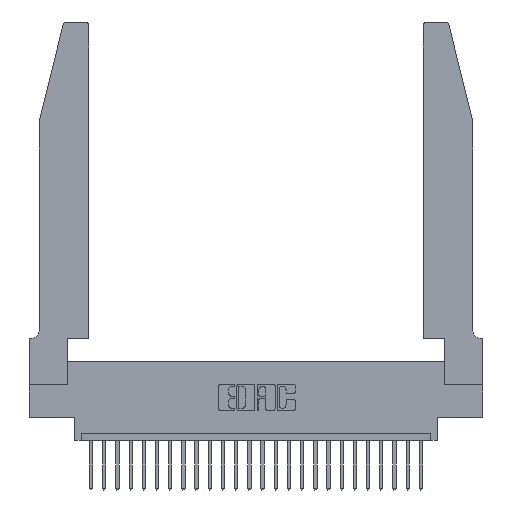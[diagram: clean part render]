
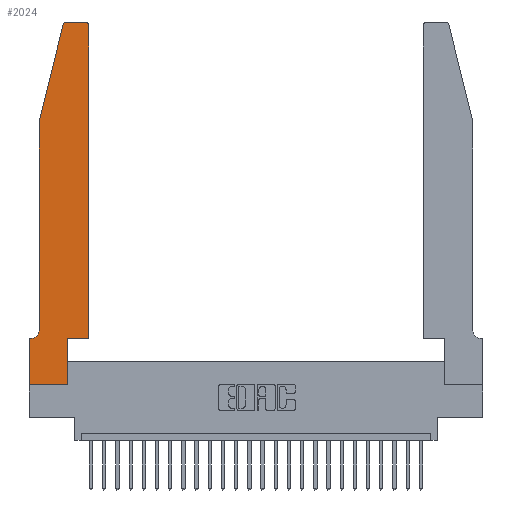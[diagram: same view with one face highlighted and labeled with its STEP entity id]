
A CAD part, top view. The second image highlights one B-rep face of the part: STEP entity #2024.
In plain terms, the highlighted planar face has unit normal (0, 0, 1).
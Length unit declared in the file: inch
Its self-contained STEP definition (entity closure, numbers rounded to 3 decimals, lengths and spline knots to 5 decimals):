
#787 = EDGE_CURVE ( 'NONE', #14174, #3340, #11736, .T. ) ;
#948 = DIRECTION ( 'NONE',  ( -1., 0., 0. ) ) ;
#1376 = DIRECTION ( 'NONE',  ( 1., 0., 0. ) ) ;
#1404 = VERTEX_POINT ( 'NONE', #18449 ) ;
#1429 = EDGE_CURVE ( 'NONE', #3409, #15677, #10569, .T. ) ;
#1465 = CIRCLE ( 'NONE', #21558, 0.07 ) ;
#1536 = DIRECTION ( 'NONE',  ( 0., -1., 0. ) ) ;
#2024 = ADVANCED_FACE ( 'NONE', ( #20470 ), #5938, .T. ) ;
#2081 = ORIENTED_EDGE ( 'NONE', *, *, #1429, .T. ) ;
#2490 = CARTESIAN_POINT ( 'NONE',  ( 0.2865, 0.35, 0.37 ) ) ;
#2954 = EDGE_CURVE ( 'NONE', #20707, #10282, #26242, .T. ) ;
#2961 = EDGE_CURVE ( 'NONE', #1404, #26402, #23984, .T. ) ;
#3164 = AXIS2_PLACEMENT_3D ( 'NONE', #8856, #6872, #21214 ) ;
#3340 = VERTEX_POINT ( 'NONE', #10819 ) ;
#3409 = VERTEX_POINT ( 'NONE', #19411 ) ;
#3444 = LINE ( 'NONE', #25226, #24611 ) ;
#3613 = EDGE_CURVE ( 'NONE', #10282, #20843, #3444, .T. ) ;
#3735 = ORIENTED_EDGE ( 'NONE', *, *, #4351, .T. ) ;
#3754 = VECTOR ( 'NONE', #24382, 39.37008 ) ;
#3763 = ORIENTED_EDGE ( 'NONE', *, *, #14501, .T. ) ;
#3949 = DIRECTION ( 'NONE',  ( 1., 0., 0. ) ) ;
#4347 = VERTEX_POINT ( 'NONE', #23082 ) ;
#4351 = EDGE_CURVE ( 'NONE', #20843, #3409, #5001, .T. ) ;
#4552 = DIRECTION ( 'NONE',  ( 0., 1., 0. ) ) ;
#5001 = LINE ( 'NONE', #21393, #19768 ) ;
#5045 = DIRECTION ( 'NONE',  ( -1., 0., 0. ) ) ;
#5938 = PLANE ( 'NONE',  #10742 ) ;
#6380 = CIRCLE ( 'NONE', #23471, 0.03 ) ;
#6781 = CARTESIAN_POINT ( 'NONE',  ( 0.0755, 0.35, 0.37 ) ) ;
#6872 = DIRECTION ( 'NONE',  ( 0., 0., 1. ) ) ;
#7204 = ORIENTED_EDGE ( 'NONE', *, *, #15792, .T. ) ;
#8226 = VECTOR ( 'NONE', #948, 39.37008 ) ;
#8350 = VERTEX_POINT ( 'NONE', #10346 ) ;
#8856 = CARTESIAN_POINT ( 'NONE',  ( 0.4205, 2.72, 0.37 ) ) ;
#10282 = VERTEX_POINT ( 'NONE', #19364 ) ;
#10346 = CARTESIAN_POINT ( 'NONE',  ( 0.284, 2.75, 0.37 ) ) ;
#10569 = LINE ( 'NONE', #2490, #11249 ) ;
#10742 = AXIS2_PLACEMENT_3D ( 'NONE', #16508, #18224, #3949 ) ;
#10819 = CARTESIAN_POINT ( 'NONE',  ( 0.0755, 0.42, 0.37 ) ) ;
#11159 = DIRECTION ( 'NONE',  ( 0., -1., 0. ) ) ;
#11249 = VECTOR ( 'NONE', #4552, 39.37008 ) ;
#11252 = CARTESIAN_POINT ( 'NONE',  ( 0.2865, 0.35, 0.37 ) ) ;
#11599 = DIRECTION ( 'NONE',  ( -0.239, -0.971, 0. ) ) ;
#11736 = LINE ( 'NONE', #19473, #17808 ) ;
#11814 = ORIENTED_EDGE ( 'NONE', *, *, #2961, .T. ) ;
#11885 = EDGE_CURVE ( 'NONE', #15677, #24329, #20150, .T. ) ;
#12162 = ORIENTED_EDGE ( 'NONE', *, *, #787, .T. ) ;
#12865 = CARTESIAN_POINT ( 'NONE',  ( 0.0055, 0.42, 0.37 ) ) ;
#13418 = VECTOR ( 'NONE', #11599, 39.37008 ) ;
#14174 = VERTEX_POINT ( 'NONE', #14208 ) ;
#14203 = EDGE_CURVE ( 'NONE', #3340, #20707, #1465, .T. ) ;
#14208 = CARTESIAN_POINT ( 'NONE',  ( 0.0755, 2., 0.37 ) ) ;
#14263 = VECTOR ( 'NONE', #21679, 39.37008 ) ;
#14501 = EDGE_CURVE ( 'NONE', #26402, #8350, #15268, .T. ) ;
#14611 = VECTOR ( 'NONE', #15788, 39.37008 ) ;
#14901 = DIRECTION ( 'NONE',  ( 0., 0., -1. ) ) ;
#15070 = ORIENTED_EDGE ( 'NONE', *, *, #3613, .T. ) ;
#15268 = LINE ( 'NONE', #15889, #14611 ) ;
#15499 = CARTESIAN_POINT ( 'NONE',  ( 0.4505, 0.35, 0.37 ) ) ;
#15677 = VERTEX_POINT ( 'NONE', #11252 ) ;
#15788 = DIRECTION ( 'NONE',  ( -1., 0., 0. ) ) ;
#15790 = ORIENTED_EDGE ( 'NONE', *, *, #11885, .T. ) ;
#15792 = EDGE_CURVE ( 'NONE', #24329, #1404, #25202, .T. ) ;
#15889 = CARTESIAN_POINT ( 'NONE',  ( 0.2605, 2.75, 0.37 ) ) ;
#15955 = CARTESIAN_POINT ( 'NONE',  ( 0.4505, 0.35, 0.37 ) ) ;
#16143 = ORIENTED_EDGE ( 'NONE', *, *, #2954, .T. ) ;
#16508 = CARTESIAN_POINT ( 'NONE',  ( 0., 0.35, 0.37 ) ) ;
#16663 = CARTESIAN_POINT ( 'NONE',  ( 0.284, 2.72, 0.37 ) ) ;
#17498 = CARTESIAN_POINT ( 'NONE',  ( 0.0755, 2., 0.37 ) ) ;
#17808 = VECTOR ( 'NONE', #11159, 39.37008 ) ;
#18224 = DIRECTION ( 'NONE',  ( 0., 0., 1. ) ) ;
#18352 = DIRECTION ( 'NONE',  ( 1., 0., 0. ) ) ;
#18442 = DIRECTION ( 'NONE',  ( 0., 0., 1. ) ) ;
#18449 = CARTESIAN_POINT ( 'NONE',  ( 0.4505, 2.72, 0.37 ) ) ;
#19364 = CARTESIAN_POINT ( 'NONE',  ( 0., 0.35, 0.37 ) ) ;
#19411 = CARTESIAN_POINT ( 'NONE',  ( 0.2865, 0., 0.37 ) ) ;
#19442 = CARTESIAN_POINT ( 'NONE',  ( 0.0055, 0.35, 0.37 ) ) ;
#19473 = CARTESIAN_POINT ( 'NONE',  ( 0.0755, 2., 0.37 ) ) ;
#19768 = VECTOR ( 'NONE', #1376, 39.37008 ) ;
#19994 = ORIENTED_EDGE ( 'NONE', *, *, #20202, .T. ) ;
#20150 = LINE ( 'NONE', #15955, #3754 ) ;
#20202 = EDGE_CURVE ( 'NONE', #4347, #14174, #23988, .T. ) ;
#20470 = FACE_OUTER_BOUND ( 'NONE', #24668, .T. ) ;
#20707 = VERTEX_POINT ( 'NONE', #19442 ) ;
#20843 = VERTEX_POINT ( 'NONE', #21652 ) ;
#21214 = DIRECTION ( 'NONE',  ( 1., 0., 0. ) ) ;
#21393 = CARTESIAN_POINT ( 'NONE',  ( 0., 0., 0.37 ) ) ;
#21558 = AXIS2_PLACEMENT_3D ( 'NONE', #12865, #14901, #5045 ) ;
#21652 = CARTESIAN_POINT ( 'NONE',  ( 0., 0., 0.37 ) ) ;
#21679 = DIRECTION ( 'NONE',  ( 0., 1., 0. ) ) ;
#23082 = CARTESIAN_POINT ( 'NONE',  ( 0.25487, 2.72718, 0.37 ) ) ;
#23471 = AXIS2_PLACEMENT_3D ( 'NONE', #16663, #18442, #18352 ) ;
#23984 = CIRCLE ( 'NONE', #3164, 0.03 ) ;
#23988 = LINE ( 'NONE', #17498, #13418 ) ;
#23998 = CARTESIAN_POINT ( 'NONE',  ( 0.4205, 2.75, 0.37 ) ) ;
#24153 = ORIENTED_EDGE ( 'NONE', *, *, #25402, .T. ) ;
#24329 = VERTEX_POINT ( 'NONE', #25032 ) ;
#24382 = DIRECTION ( 'NONE',  ( 1., 0., 0. ) ) ;
#24611 = VECTOR ( 'NONE', #1536, 39.37008 ) ;
#24668 = EDGE_LOOP ( 'NONE', ( #3763, #24153, #19994, #12162, #25526, #16143, #15070, #3735, #2081, #15790, #7204, #11814 ) ) ;
#25032 = CARTESIAN_POINT ( 'NONE',  ( 0.4505, 0.35, 0.37 ) ) ;
#25202 = LINE ( 'NONE', #15499, #14263 ) ;
#25226 = CARTESIAN_POINT ( 'NONE',  ( 0., 0., 0.37 ) ) ;
#25402 = EDGE_CURVE ( 'NONE', #8350, #4347, #6380, .T. ) ;
#25526 = ORIENTED_EDGE ( 'NONE', *, *, #14203, .T. ) ;
#26242 = LINE ( 'NONE', #6781, #8226 ) ;
#26402 = VERTEX_POINT ( 'NONE', #23998 ) ;
